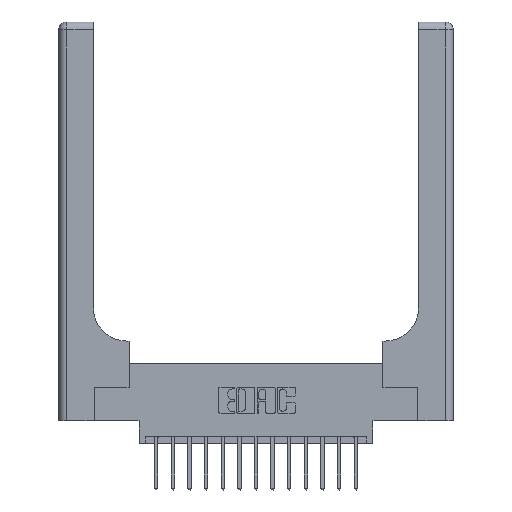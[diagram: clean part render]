
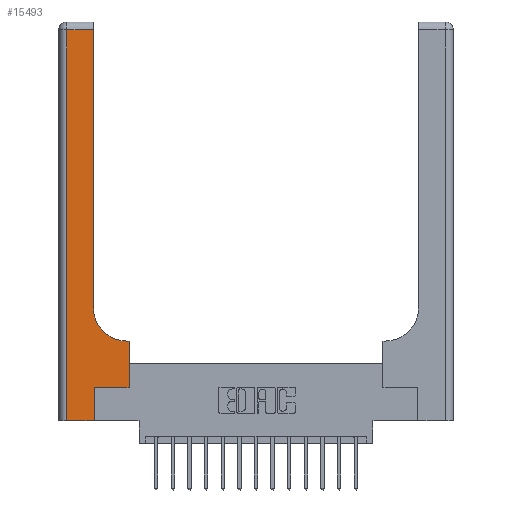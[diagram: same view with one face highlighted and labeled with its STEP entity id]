
A CAD part, top view. The second image highlights one B-rep face of the part: STEP entity #15493.
In plain terms, the highlighted planar face has unit normal (0, 0, 1).
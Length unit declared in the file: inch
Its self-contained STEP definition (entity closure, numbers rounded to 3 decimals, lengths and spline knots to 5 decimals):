
#404 = CARTESIAN_POINT ( 'NONE',  ( 0.265, 0., 0.37 ) ) ;
#487 = DIRECTION ( 'NONE',  ( -1., 0., 0. ) ) ;
#1404 = VERTEX_POINT ( 'NONE', #2895 ) ;
#1494 = EDGE_LOOP ( 'NONE', ( #17102, #17541, #7097, #11174, #4711, #15624, #1901, #9244, #9690 ) ) ;
#1530 = DIRECTION ( 'NONE',  ( -1., 0., 0. ) ) ;
#1603 = CARTESIAN_POINT ( 'NONE',  ( 0.06, 2.94, 0.37 ) ) ;
#1724 = AXIS2_PLACEMENT_3D ( 'NONE', #4722, #10308, #2065 ) ;
#1901 = ORIENTED_EDGE ( 'NONE', *, *, #10408, .T. ) ;
#2065 = DIRECTION ( 'NONE',  ( -1., 0., 0. ) ) ;
#2272 = AXIS2_PLACEMENT_3D ( 'NONE', #14453, #6252, #15805 ) ;
#2350 = DIRECTION ( 'NONE',  ( 0., -1., 0. ) ) ;
#2816 = EDGE_CURVE ( 'NONE', #9834, #5765, #6068, .T. ) ;
#2895 = CARTESIAN_POINT ( 'NONE',  ( 0.26, 0.85, 0.37 ) ) ;
#3451 = CARTESIAN_POINT ( 'NONE',  ( 0.528, 0.6, 0.37 ) ) ;
#3614 = CARTESIAN_POINT ( 'NONE',  ( 0.528, 0.25, 0.37 ) ) ;
#3615 = DIRECTION ( 'NONE',  ( 1., 0., 0. ) ) ;
#3961 = CARTESIAN_POINT ( 'NONE',  ( 0.265, 0.25, 0.37 ) ) ;
#4187 = DIRECTION ( 'NONE',  ( 0., 1., 0. ) ) ;
#4583 = LINE ( 'NONE', #16208, #11904 ) ;
#4711 = ORIENTED_EDGE ( 'NONE', *, *, #2816, .T. ) ;
#4722 = CARTESIAN_POINT ( 'NONE',  ( 0., 3., 0.37 ) ) ;
#4872 = FACE_OUTER_BOUND ( 'NONE', #1494, .T. ) ;
#4887 = DIRECTION ( 'NONE',  ( 1., 0., 0. ) ) ;
#5276 = DIRECTION ( 'NONE',  ( 0., 1., 0. ) ) ;
#5765 = VERTEX_POINT ( 'NONE', #3961 ) ;
#6011 = CIRCLE ( 'NONE', #2272, 0.25 ) ;
#6068 = LINE ( 'NONE', #15208, #9307 ) ;
#6252 = DIRECTION ( 'NONE',  ( 0., 0., -1. ) ) ;
#7097 = ORIENTED_EDGE ( 'NONE', *, *, #15922, .T. ) ;
#7469 = CARTESIAN_POINT ( 'NONE',  ( 0.26, 2.94, 0.37 ) ) ;
#7511 = VERTEX_POINT ( 'NONE', #16836 ) ;
#7988 = EDGE_CURVE ( 'NONE', #1404, #11485, #11509, .T. ) ;
#8025 = LINE ( 'NONE', #11980, #15703 ) ;
#8435 = CARTESIAN_POINT ( 'NONE',  ( 0.26, 3., 0.37 ) ) ;
#8745 = CARTESIAN_POINT ( 'NONE',  ( 0., 2.94, 0.37 ) ) ;
#9151 = CARTESIAN_POINT ( 'NONE',  ( 0.06, 0., 0.37 ) ) ;
#9244 = ORIENTED_EDGE ( 'NONE', *, *, #17356, .T. ) ;
#9307 = VECTOR ( 'NONE', #4187, 39.37008 ) ;
#9325 = VECTOR ( 'NONE', #4887, 39.37008 ) ;
#9690 = ORIENTED_EDGE ( 'NONE', *, *, #13049, .T. ) ;
#9834 = VERTEX_POINT ( 'NONE', #404 ) ;
#9925 = LINE ( 'NONE', #8745, #10326 ) ;
#10133 = LINE ( 'NONE', #16560, #16079 ) ;
#10308 = DIRECTION ( 'NONE',  ( 0., 0., -1. ) ) ;
#10326 = VECTOR ( 'NONE', #487, 39.37008 ) ;
#10408 = EDGE_CURVE ( 'NONE', #17722, #15516, #4583, .T. ) ;
#10479 = LINE ( 'NONE', #13218, #17284 ) ;
#11174 = ORIENTED_EDGE ( 'NONE', *, *, #14373, .T. ) ;
#11485 = VERTEX_POINT ( 'NONE', #7469 ) ;
#11509 = LINE ( 'NONE', #8435, #15118 ) ;
#11540 = VERTEX_POINT ( 'NONE', #9151 ) ;
#11904 = VECTOR ( 'NONE', #5276, 39.37008 ) ;
#11980 = CARTESIAN_POINT ( 'NONE',  ( 0.06, 3., 0.37 ) ) ;
#13049 = EDGE_CURVE ( 'NONE', #7511, #1404, #6011, .T. ) ;
#13102 = CARTESIAN_POINT ( 'NONE',  ( 0.265, 0.25, 0.37 ) ) ;
#13218 = CARTESIAN_POINT ( 'NONE',  ( 0., 0., 0.37 ) ) ;
#14363 = PLANE ( 'NONE',  #1724 ) ;
#14373 = EDGE_CURVE ( 'NONE', #11540, #9834, #10479, .T. ) ;
#14453 = CARTESIAN_POINT ( 'NONE',  ( 0.51, 0.85, 0.37 ) ) ;
#15118 = VECTOR ( 'NONE', #16593, 39.37008 ) ;
#15208 = CARTESIAN_POINT ( 'NONE',  ( 0.265, 0., 0.37 ) ) ;
#15329 = VERTEX_POINT ( 'NONE', #1603 ) ;
#15493 = ADVANCED_FACE ( 'NONE', ( #4872 ), #14363, .F. ) ;
#15516 = VERTEX_POINT ( 'NONE', #3451 ) ;
#15624 = ORIENTED_EDGE ( 'NONE', *, *, #15829, .T. ) ;
#15703 = VECTOR ( 'NONE', #2350, 39.37008 ) ;
#15805 = DIRECTION ( 'NONE',  ( 1., 0., 0. ) ) ;
#15829 = EDGE_CURVE ( 'NONE', #5765, #17722, #16131, .T. ) ;
#15922 = EDGE_CURVE ( 'NONE', #15329, #11540, #8025, .T. ) ;
#16079 = VECTOR ( 'NONE', #1530, 39.37008 ) ;
#16131 = LINE ( 'NONE', #13102, #9325 ) ;
#16208 = CARTESIAN_POINT ( 'NONE',  ( 0.528, 0.25, 0.37 ) ) ;
#16560 = CARTESIAN_POINT ( 'NONE',  ( 0.26, 0.6, 0.37 ) ) ;
#16593 = DIRECTION ( 'NONE',  ( 0., 1., 0. ) ) ;
#16836 = CARTESIAN_POINT ( 'NONE',  ( 0.51, 0.6, 0.37 ) ) ;
#17102 = ORIENTED_EDGE ( 'NONE', *, *, #7988, .T. ) ;
#17284 = VECTOR ( 'NONE', #3615, 39.37008 ) ;
#17356 = EDGE_CURVE ( 'NONE', #15516, #7511, #10133, .T. ) ;
#17520 = EDGE_CURVE ( 'NONE', #11485, #15329, #9925, .T. ) ;
#17541 = ORIENTED_EDGE ( 'NONE', *, *, #17520, .T. ) ;
#17722 = VERTEX_POINT ( 'NONE', #3614 ) ;
